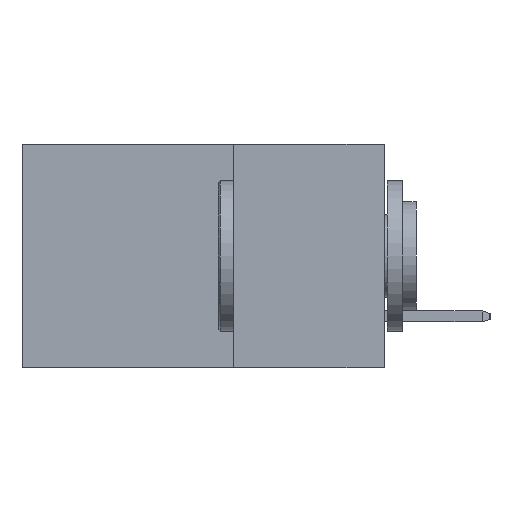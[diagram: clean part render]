
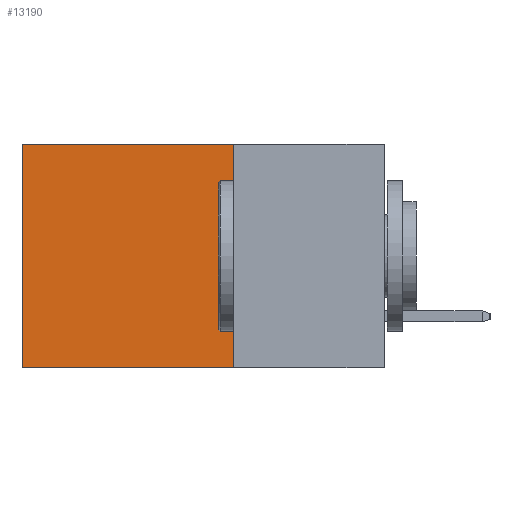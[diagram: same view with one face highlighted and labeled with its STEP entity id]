
A CAD part, left-side view. The second image highlights one B-rep face of the part: STEP entity #13190.
In plain terms, the highlighted planar face has unit normal (-1, 0, 0).
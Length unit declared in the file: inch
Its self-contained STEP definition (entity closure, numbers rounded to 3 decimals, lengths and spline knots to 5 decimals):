
#179 = CARTESIAN_POINT ( 'NONE',  ( 0.298, 0.6, 0. ) ) ;
#295 = LINE ( 'NONE', #17779, #7982 ) ;
#1917 = CARTESIAN_POINT ( 'NONE',  ( 0.298, 0.25, 0. ) ) ;
#2532 = VECTOR ( 'NONE', #6152, 39.37008 ) ;
#2559 = CARTESIAN_POINT ( 'NONE',  ( 0.298, 0.25, 0. ) ) ;
#2977 = LINE ( 'NONE', #12597, #10124 ) ;
#3462 = DIRECTION ( 'NONE',  ( 1., 0., 0. ) ) ;
#4735 = CARTESIAN_POINT ( 'NONE',  ( 0.298, 0.25, 0. ) ) ;
#4991 = EDGE_CURVE ( 'NONE', #6494, #10195, #2977, .T. ) ;
#5215 = ORIENTED_EDGE ( 'NONE', *, *, #10688, .F. ) ;
#6152 = DIRECTION ( 'NONE',  ( 0., 0., -1. ) ) ;
#6494 = VERTEX_POINT ( 'NONE', #179 ) ;
#7982 = VECTOR ( 'NONE', #14745, 39.37008 ) ;
#8040 = ORIENTED_EDGE ( 'NONE', *, *, #18506, .T. ) ;
#8043 = VERTEX_POINT ( 'NONE', #2559 ) ;
#8642 = ORIENTED_EDGE ( 'NONE', *, *, #4991, .T. ) ;
#9591 = DIRECTION ( 'NONE',  ( 0., 0., -1. ) ) ;
#10124 = VECTOR ( 'NONE', #9591, 39.37008 ) ;
#10195 = VERTEX_POINT ( 'NONE', #18503 ) ;
#10688 = EDGE_CURVE ( 'NONE', #8043, #16261, #11094, .T. ) ;
#11029 = PLANE ( 'NONE',  #12224 ) ;
#11094 = LINE ( 'NONE', #13671, #2532 ) ;
#12014 = DIRECTION ( 'NONE',  ( 0., 1., 0. ) ) ;
#12224 = AXIS2_PLACEMENT_3D ( 'NONE', #1917, #3462, #14069 ) ;
#12597 = CARTESIAN_POINT ( 'NONE',  ( 0.298, 0.6, 0. ) ) ;
#13190 = ADVANCED_FACE ( 'NONE', ( #17826 ), #11029, .F. ) ;
#13443 = ORIENTED_EDGE ( 'NONE', *, *, #18035, .F. ) ;
#13671 = CARTESIAN_POINT ( 'NONE',  ( 0.298, 0.25, 0. ) ) ;
#14069 = DIRECTION ( 'NONE',  ( 0., 0., -1. ) ) ;
#14745 = DIRECTION ( 'NONE',  ( 0., 1., 0. ) ) ;
#15064 = LINE ( 'NONE', #4735, #19027 ) ;
#16261 = VERTEX_POINT ( 'NONE', #17173 ) ;
#17173 = CARTESIAN_POINT ( 'NONE',  ( 0.298, 0.25, -0.37 ) ) ;
#17765 = EDGE_LOOP ( 'NONE', ( #8642, #13443, #5215, #8040 ) ) ;
#17779 = CARTESIAN_POINT ( 'NONE',  ( 0.298, 0.25, -0.37 ) ) ;
#17826 = FACE_OUTER_BOUND ( 'NONE', #17765, .T. ) ;
#18035 = EDGE_CURVE ( 'NONE', #16261, #10195, #295, .T. ) ;
#18503 = CARTESIAN_POINT ( 'NONE',  ( 0.298, 0.6, -0.37 ) ) ;
#18506 = EDGE_CURVE ( 'NONE', #8043, #6494, #15064, .T. ) ;
#19027 = VECTOR ( 'NONE', #12014, 39.37008 ) ;
